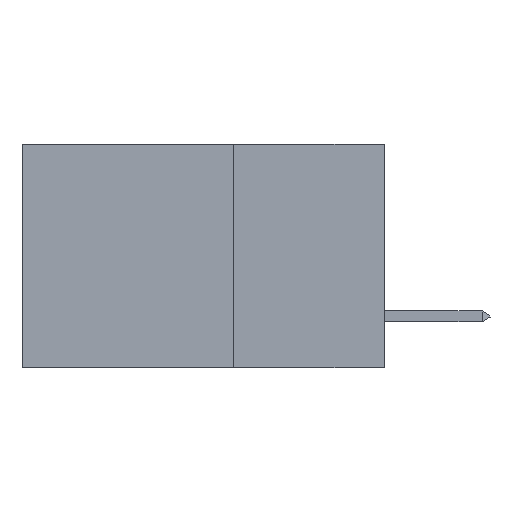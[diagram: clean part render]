
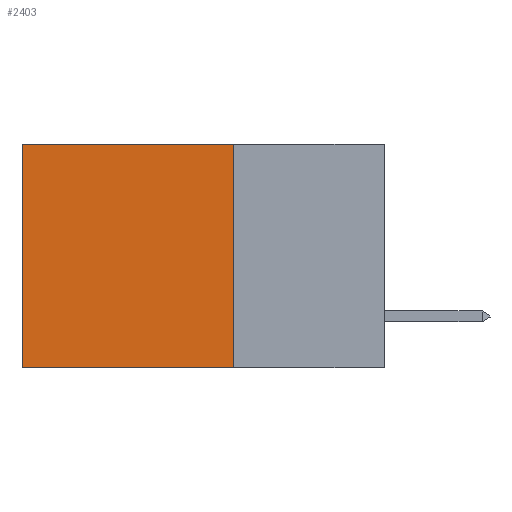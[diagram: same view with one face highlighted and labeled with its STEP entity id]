
A CAD part, left-side view. The second image highlights one B-rep face of the part: STEP entity #2403.
In plain terms, the highlighted planar face has unit normal (-1, 0, 0).
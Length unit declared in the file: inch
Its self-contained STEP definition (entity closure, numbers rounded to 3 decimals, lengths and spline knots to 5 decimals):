
#864 = VECTOR ( 'NONE', #21609, 39.37008 ) ;
#1828 = EDGE_CURVE ( 'NONE', #10212, #11674, #27561, .T. ) ;
#1979 = DIRECTION ( 'NONE',  ( 1., 0., 0. ) ) ;
#2403 = ADVANCED_FACE ( 'NONE', ( #5438 ), #28375, .F. ) ;
#2956 = DIRECTION ( 'NONE',  ( 0., 1., 0. ) ) ;
#3080 = ORIENTED_EDGE ( 'NONE', *, *, #25104, .T. ) ;
#3642 = LINE ( 'NONE', #13056, #864 ) ;
#5079 = CARTESIAN_POINT ( 'NONE',  ( 0.2875, 0.25, 0. ) ) ;
#5438 = FACE_OUTER_BOUND ( 'NONE', #21491, .T. ) ;
#5521 = CARTESIAN_POINT ( 'NONE',  ( 0.2875, 0.25, 0. ) ) ;
#7826 = ORIENTED_EDGE ( 'NONE', *, *, #21219, .F. ) ;
#7922 = VECTOR ( 'NONE', #2956, 39.37008 ) ;
#7981 = CARTESIAN_POINT ( 'NONE',  ( 0.2875, 0.6, 0. ) ) ;
#9631 = ORIENTED_EDGE ( 'NONE', *, *, #1828, .T. ) ;
#10212 = VERTEX_POINT ( 'NONE', #5521 ) ;
#10734 = DIRECTION ( 'NONE',  ( 0., 1., 0. ) ) ;
#10760 = VECTOR ( 'NONE', #10734, 39.37008 ) ;
#11674 = VERTEX_POINT ( 'NONE', #7981 ) ;
#12474 = LINE ( 'NONE', #17659, #10760 ) ;
#12875 = VERTEX_POINT ( 'NONE', #19435 ) ;
#12889 = ORIENTED_EDGE ( 'NONE', *, *, #19240, .F. ) ;
#13056 = CARTESIAN_POINT ( 'NONE',  ( 0.2875, 0.6, 0. ) ) ;
#13819 = CARTESIAN_POINT ( 'NONE',  ( 0.2875, 0.25, 0. ) ) ;
#15184 = CARTESIAN_POINT ( 'NONE',  ( 0.2875, 0.25, 0. ) ) ;
#17379 = DIRECTION ( 'NONE',  ( 0., 0., -1. ) ) ;
#17659 = CARTESIAN_POINT ( 'NONE',  ( 0.2875, 0.25, -0.37 ) ) ;
#17845 = DIRECTION ( 'NONE',  ( 0., 0., -1. ) ) ;
#18117 = LINE ( 'NONE', #13819, #27928 ) ;
#19240 = EDGE_CURVE ( 'NONE', #10212, #12875, #18117, .T. ) ;
#19435 = CARTESIAN_POINT ( 'NONE',  ( 0.2875, 0.25, -0.37 ) ) ;
#19726 = AXIS2_PLACEMENT_3D ( 'NONE', #15184, #1979, #17379 ) ;
#21219 = EDGE_CURVE ( 'NONE', #12875, #25892, #12474, .T. ) ;
#21491 = EDGE_LOOP ( 'NONE', ( #3080, #7826, #12889, #9631 ) ) ;
#21609 = DIRECTION ( 'NONE',  ( 0., 0., -1. ) ) ;
#25104 = EDGE_CURVE ( 'NONE', #11674, #25892, #3642, .T. ) ;
#25892 = VERTEX_POINT ( 'NONE', #27999 ) ;
#27561 = LINE ( 'NONE', #5079, #7922 ) ;
#27928 = VECTOR ( 'NONE', #17845, 39.37008 ) ;
#27999 = CARTESIAN_POINT ( 'NONE',  ( 0.2875, 0.6, -0.37 ) ) ;
#28375 = PLANE ( 'NONE',  #19726 ) ;
